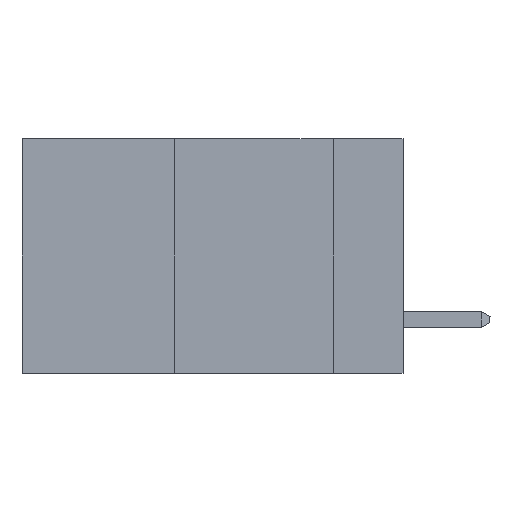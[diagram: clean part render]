
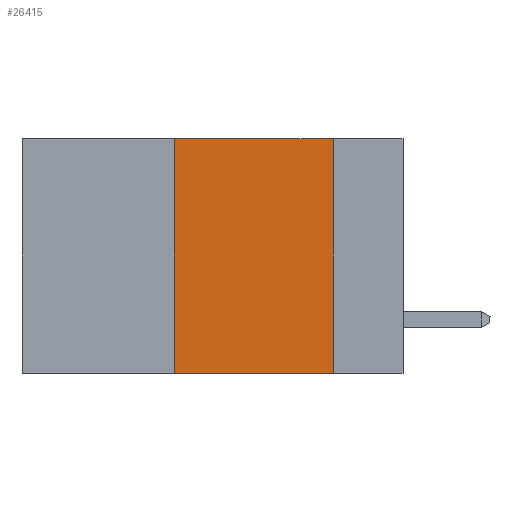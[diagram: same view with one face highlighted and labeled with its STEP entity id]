
A CAD part, left-side view. The second image highlights one B-rep face of the part: STEP entity #26415.
In plain terms, the highlighted planar face has unit normal (-1, 0, 0).
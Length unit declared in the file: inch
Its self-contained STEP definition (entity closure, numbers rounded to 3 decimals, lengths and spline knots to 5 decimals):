
#37 = VERTEX_POINT ( 'NONE', #21223 ) ;
#57 = ORIENTED_EDGE ( 'NONE', *, *, #15017, .F. ) ;
#537 = LINE ( 'NONE', #20284, #18531 ) ;
#629 = PLANE ( 'NONE',  #35777 ) ;
#1070 = EDGE_CURVE ( 'NONE', #37, #35337, #17231, .T. ) ;
#2580 = VECTOR ( 'NONE', #7389, 39.37008 ) ;
#7085 = ORIENTED_EDGE ( 'NONE', *, *, #15389, .F. ) ;
#7252 = VERTEX_POINT ( 'NONE', #31262 ) ;
#7389 = DIRECTION ( 'NONE',  ( 0., 0., 1. ) ) ;
#8763 = DIRECTION ( 'NONE',  ( 1., 0., 0. ) ) ;
#12212 = EDGE_LOOP ( 'NONE', ( #27736, #7085, #57, #35121 ) ) ;
#15017 = EDGE_CURVE ( 'NONE', #7252, #26590, #34554, .T. ) ;
#15389 = EDGE_CURVE ( 'NONE', #26590, #37, #537, .T. ) ;
#16896 = FACE_OUTER_BOUND ( 'NONE', #12212, .T. ) ;
#17231 = LINE ( 'NONE', #25525, #27015 ) ;
#18531 = VECTOR ( 'NONE', #34696, 39.37008 ) ;
#18630 = CARTESIAN_POINT ( 'NONE',  ( 0., 0.6, -0.37 ) ) ;
#18851 = CARTESIAN_POINT ( 'NONE',  ( 0., 0.36, 0. ) ) ;
#20284 = CARTESIAN_POINT ( 'NONE',  ( 0., 0.6, 0. ) ) ;
#21223 = CARTESIAN_POINT ( 'NONE',  ( 0., 0.11, 0. ) ) ;
#22426 = CARTESIAN_POINT ( 'NONE',  ( 0., 0.6, 0. ) ) ;
#23791 = LINE ( 'NONE', #18630, #32568 ) ;
#25525 = CARTESIAN_POINT ( 'NONE',  ( 0., 0.11, 0. ) ) ;
#26415 = ADVANCED_FACE ( 'NONE', ( #16896 ), #629, .F. ) ;
#26470 = CARTESIAN_POINT ( 'NONE',  ( 0., 0.36, 0. ) ) ;
#26590 = VERTEX_POINT ( 'NONE', #26470 ) ;
#26746 = DIRECTION ( 'NONE',  ( 0., -1., 0. ) ) ;
#27015 = VECTOR ( 'NONE', #29022, 39.37008 ) ;
#27736 = ORIENTED_EDGE ( 'NONE', *, *, #1070, .F. ) ;
#28154 = DIRECTION ( 'NONE',  ( 0., 0., -1. ) ) ;
#29022 = DIRECTION ( 'NONE',  ( 0., 0., -1. ) ) ;
#31262 = CARTESIAN_POINT ( 'NONE',  ( 0., 0.36, -0.37 ) ) ;
#31357 = CARTESIAN_POINT ( 'NONE',  ( 0., 0.11, -0.37 ) ) ;
#31805 = EDGE_CURVE ( 'NONE', #7252, #35337, #23791, .T. ) ;
#32568 = VECTOR ( 'NONE', #26746, 39.37008 ) ;
#34554 = LINE ( 'NONE', #18851, #2580 ) ;
#34696 = DIRECTION ( 'NONE',  ( 0., -1., 0. ) ) ;
#35121 = ORIENTED_EDGE ( 'NONE', *, *, #31805, .T. ) ;
#35337 = VERTEX_POINT ( 'NONE', #31357 ) ;
#35777 = AXIS2_PLACEMENT_3D ( 'NONE', #22426, #8763, #28154 ) ;
